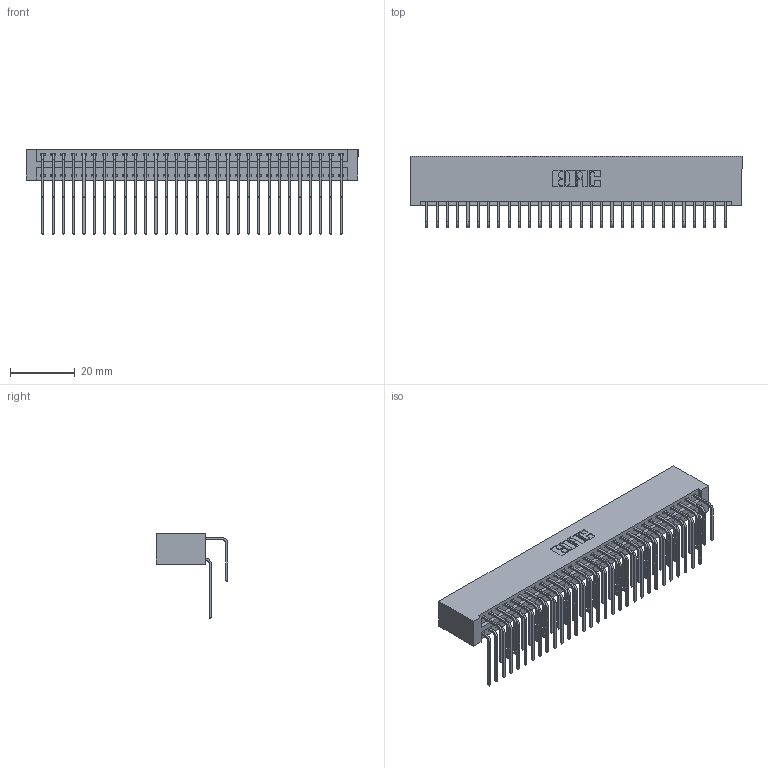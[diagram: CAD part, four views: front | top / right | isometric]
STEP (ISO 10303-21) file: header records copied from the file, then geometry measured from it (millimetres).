
FILE_DESCRIPTION (( 'STEP AP203' ), '1' );
FILE_NAME ('346-060-558-201.STEP', '2018-08-28T06:15:16', ( '' ), ( '' ), 'SwSTEP 2.0', 'SolidWorks 2016', '' );
FILE_SCHEMA (( 'CONFIG_CONTROL_DESIGN' ));
Length unit declared in the file: inch
Products named in the file (4): 345-292-001_558 Tail - 2; 346-060-558-201; 346 Part_No Mounting Lugs; 345-292-001_558 559 Tail - 1
Assembly tree (61 placements, depth 2):
  346-060-558-201
    346 Part_No Mounting Lugs
    345-292-001_558 559 Tail - 1  x30
    345-292-001_558 Tail - 2  x30
Bounding box: 102.49 x 22.16 x 26.16 mm (x, y, z)
Volume: 10820.2 mm3; surface area: 16508.1 mm2
Topology: 61 solids, 61 shells, 3354 faces, 9965 edges, 6562 vertices
Faces by surface type: plane 2292, cylinder 1062
Entity records: 22701 total; most frequent: CARTESIAN_POINT 3807, ORIENTED_EDGE 3690, DIRECTION 3373, EDGE_CURVE 1845, VECTOR 1561, LINE 1561, VERTEX_POINT 1226, AXIS2_PLACEMENT_3D 906
